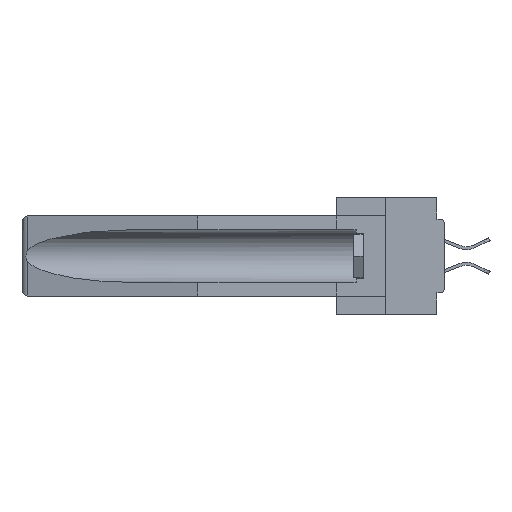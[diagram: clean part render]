
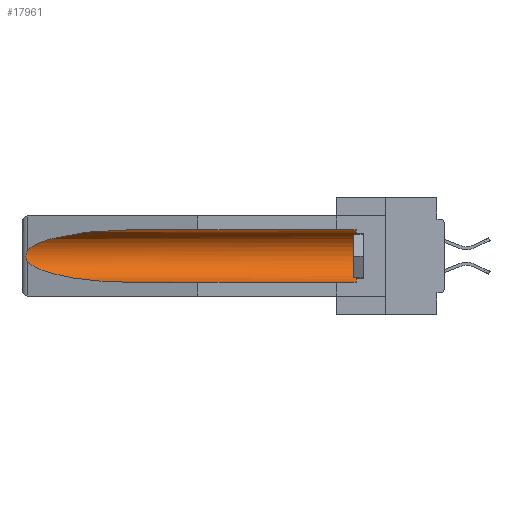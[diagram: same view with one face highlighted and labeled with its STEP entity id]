
A CAD part, left-side view. The second image highlights one B-rep face of the part: STEP entity #17961.
In plain terms, the highlighted cylindrical face has radius 2.857 mm (diameter 5.715 mm), a partial arc.
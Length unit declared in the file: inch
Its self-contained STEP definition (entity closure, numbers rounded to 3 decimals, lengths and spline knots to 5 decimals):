
#1717 = CARTESIAN_POINT ( 'NONE',  ( 0.26537, 1.52718, -0.19328 ) ) ;
#2749 = CARTESIAN_POINT ( 'NONE',  ( 0.26655, 1.53094, -0.18657 ) ) ;
#4660 = DIRECTION ( 'NONE',  ( 0., 1., 0. ) ) ;
#5776 = EDGE_CURVE ( 'NONE', #42004, #25340, #13097, .T. ) ;
#6226 = CARTESIAN_POINT ( 'NONE',  ( 0.155, -0.30754, -0.059 ) ) ;
#6252 = DIRECTION ( 'NONE',  ( 0., -1., 0. ) ) ;
#6761 = CYLINDRICAL_SURFACE ( 'NONE', #10258, 0.1125 ) ;
#8139 = CARTESIAN_POINT ( 'NONE',  ( 0.155, -0.30754, -0.284 ) ) ;
#8641 = ORIENTED_EDGE ( 'NONE', *, *, #22271, .T. ) ;
#8693 = CARTESIAN_POINT ( 'NONE',  ( 0.21114, 1.30732, -0.059 ) ) ;
#9000 = CARTESIAN_POINT ( 'NONE',  ( 0.26537, 1.52718, -0.14972 ) ) ;
#10004 = DIRECTION ( 'NONE',  ( 0., 1., 0. ) ) ;
#10258 = AXIS2_PLACEMENT_3D ( 'NONE', #44629, #23266, #33434 ) ;
#12610 = CARTESIAN_POINT ( 'NONE',  ( 0.25451, 1.48313, -0.09465 ) ) ;
#12813 = CARTESIAN_POINT ( 'NONE',  ( 0.155, 1.07973, -0.284 ) ) ;
#13097 =( BOUNDED_CURVE ( )  B_SPLINE_CURVE ( 3, ( #1717, #16051, #19470, #12813 ),
 .UNSPECIFIED., .F., .T. ) 
 B_SPLINE_CURVE_WITH_KNOTS ( ( 4, 4 ),
 ( 0.1948, 1.5708 ),
 .UNSPECIFIED. ) 
 CURVE ( )  GEOMETRIC_REPRESENTATION_ITEM ( )  RATIONAL_B_SPLINE_CURVE ( ( 1., 0.848, 0.848, 1. ) ) 
 REPRESENTATION_ITEM ( '' )  );
#14115 = CARTESIAN_POINT ( 'NONE',  ( 0.155, 0.126, -0.059 ) ) ;
#14452 = CIRCLE ( 'NONE', #39389, 0.1125 ) ;
#16029 = B_SPLINE_CURVE_WITH_KNOTS ( 'NONE', 3,
 ( #28036, #16933, #20832, #38772, #31632, #45318, #38608, #2749, #27712, #17245 ),
 .UNSPECIFIED., .F., .F.,
 ( 4, 2, 2, 2, 4 ),
 ( 0., 0.00029, 0.00058, 0.00087, 0.00117 ),
 .UNSPECIFIED. ) ;
#16051 = CARTESIAN_POINT ( 'NONE',  ( 0.25451, 1.48313, -0.24835 ) ) ;
#16166 = ORIENTED_EDGE ( 'NONE', *, *, #22664, .F. ) ;
#16933 = CARTESIAN_POINT ( 'NONE',  ( 0.26597, 1.52961, -0.15275 ) ) ;
#17245 = CARTESIAN_POINT ( 'NONE',  ( 0.26537, 1.52718, -0.19328 ) ) ;
#17961 = ADVANCED_FACE ( 'NONE', ( #24069 ), #6761, .F. ) ;
#19470 = CARTESIAN_POINT ( 'NONE',  ( 0.21114, 1.30732, -0.284 ) ) ;
#19511 = CARTESIAN_POINT ( 'NONE',  ( 0.155, 0.126, -0.284 ) ) ;
#19678 = ORIENTED_EDGE ( 'NONE', *, *, #26091, .T. ) ;
#20261 = VERTEX_POINT ( 'NONE', #14115 ) ;
#20742 = DIRECTION ( 'NONE',  ( 0., 0., 1. ) ) ;
#20832 = CARTESIAN_POINT ( 'NONE',  ( 0.26654, 1.53092, -0.15636 ) ) ;
#22037 = LINE ( 'NONE', #6226, #27054 ) ;
#22271 = EDGE_CURVE ( 'NONE', #42948, #45342, #32619, .T. ) ;
#22664 = EDGE_CURVE ( 'NONE', #37401, #25340, #43558, .T. ) ;
#23266 = DIRECTION ( 'NONE',  ( 0., 1., 0. ) ) ;
#23760 = ORIENTED_EDGE ( 'NONE', *, *, #37481, .T. ) ;
#24069 = FACE_OUTER_BOUND ( 'NONE', #43254, .T. ) ;
#25340 = VERTEX_POINT ( 'NONE', #44938 ) ;
#26091 = EDGE_CURVE ( 'NONE', #37401, #20261, #14452, .T. ) ;
#27054 = VECTOR ( 'NONE', #10004, 39.37008 ) ;
#27712 = CARTESIAN_POINT ( 'NONE',  ( 0.26597, 1.5296, -0.19026 ) ) ;
#28036 = CARTESIAN_POINT ( 'NONE',  ( 0.26537, 1.52718, -0.14972 ) ) ;
#28388 = CARTESIAN_POINT ( 'NONE',  ( 0.26537, 1.52718, -0.14972 ) ) ;
#31632 = CARTESIAN_POINT ( 'NONE',  ( 0.2675, 1.53308, -0.16763 ) ) ;
#32619 =( BOUNDED_CURVE ( )  B_SPLINE_CURVE ( 3, ( #33476, #8693, #12610, #9000 ),
 .UNSPECIFIED., .F., .F. ) 
 B_SPLINE_CURVE_WITH_KNOTS ( ( 4, 4 ),
 ( 4.71239, 6.08839 ),
 .UNSPECIFIED. ) 
 CURVE ( )  GEOMETRIC_REPRESENTATION_ITEM ( )  RATIONAL_B_SPLINE_CURVE ( ( 1., 0.848, 0.848, 1. ) ) 
 REPRESENTATION_ITEM ( '' )  );
#33434 = DIRECTION ( 'NONE',  ( 0., 0., 1. ) ) ;
#33476 = CARTESIAN_POINT ( 'NONE',  ( 0.155, 1.07973, -0.059 ) ) ;
#36089 = EDGE_CURVE ( 'NONE', #45342, #42004, #16029, .T. ) ;
#36403 = CARTESIAN_POINT ( 'NONE',  ( 0.155, 1.07973, -0.059 ) ) ;
#37401 = VERTEX_POINT ( 'NONE', #19511 ) ;
#37481 = EDGE_CURVE ( 'NONE', #20261, #42948, #22037, .T. ) ;
#38608 = CARTESIAN_POINT ( 'NONE',  ( 0.2673, 1.53269, -0.17917 ) ) ;
#38772 = CARTESIAN_POINT ( 'NONE',  ( 0.2673, 1.5327, -0.16383 ) ) ;
#39229 = ORIENTED_EDGE ( 'NONE', *, *, #5776, .T. ) ;
#39389 = AXIS2_PLACEMENT_3D ( 'NONE', #41832, #6252, #20742 ) ;
#41832 = CARTESIAN_POINT ( 'NONE',  ( 0.155, 0.126, -0.1715 ) ) ;
#42004 = VERTEX_POINT ( 'NONE', #45069 ) ;
#42452 = VECTOR ( 'NONE', #4660, 39.37008 ) ;
#42948 = VERTEX_POINT ( 'NONE', #36403 ) ;
#43254 = EDGE_LOOP ( 'NONE', ( #8641, #43634, #39229, #16166, #19678, #23760 ) ) ;
#43558 = LINE ( 'NONE', #8139, #42452 ) ;
#43634 = ORIENTED_EDGE ( 'NONE', *, *, #36089, .T. ) ;
#44629 = CARTESIAN_POINT ( 'NONE',  ( 0.155, -0.30754, -0.1715 ) ) ;
#44938 = CARTESIAN_POINT ( 'NONE',  ( 0.155, 1.07973, -0.284 ) ) ;
#45069 = CARTESIAN_POINT ( 'NONE',  ( 0.26537, 1.52718, -0.19328 ) ) ;
#45318 = CARTESIAN_POINT ( 'NONE',  ( 0.2675, 1.53308, -0.17534 ) ) ;
#45342 = VERTEX_POINT ( 'NONE', #28388 ) ;
